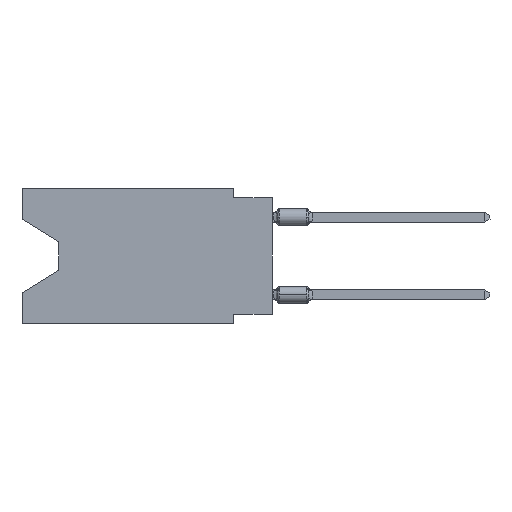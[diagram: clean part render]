
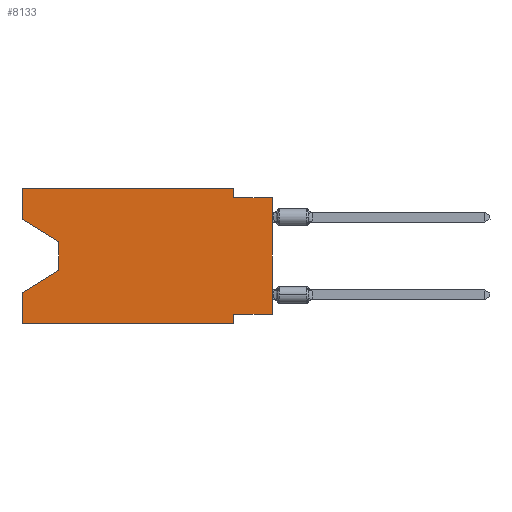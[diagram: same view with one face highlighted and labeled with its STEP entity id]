
A CAD part, left-side view. The second image highlights one B-rep face of the part: STEP entity #8133.
In plain terms, the highlighted planar face has unit normal (-1, 0, 0).
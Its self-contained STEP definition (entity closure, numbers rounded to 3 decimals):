
#111 = DIRECTION ( 'NONE',  ( 0., -1., 0. ) ) ;
#298 = DIRECTION ( 'NONE',  ( 0., 1., 0. ) ) ;
#623 = CARTESIAN_POINT ( 'NONE',  ( 0., 16.383, -2.038 ) ) ;
#681 = CARTESIAN_POINT ( 'NONE',  ( 0., 16.383, -8.89 ) ) ;
#780 = EDGE_CURVE ( 'NONE', #9780, #29481, #25678, .T. ) ;
#806 = CARTESIAN_POINT ( 'NONE',  ( 0., 0., 0. ) ) ;
#1141 = EDGE_CURVE ( 'NONE', #27086, #24400, #24019, .T. ) ;
#2260 = VECTOR ( 'NONE', #25266, 1000. ) ;
#2419 = DIRECTION ( 'NONE',  ( 1., 0., 0. ) ) ;
#2759 = CARTESIAN_POINT ( 'NONE',  ( 0., 0., -8.255 ) ) ;
#2879 = VERTEX_POINT ( 'NONE', #31622 ) ;
#2957 = DIRECTION ( 'NONE',  ( 0., -1., 0. ) ) ;
#3117 = CARTESIAN_POINT ( 'NONE',  ( 0., 16.383, -8.89 ) ) ;
#3632 = DIRECTION ( 'NONE',  ( 0., 0., -1. ) ) ;
#4514 = ORIENTED_EDGE ( 'NONE', *, *, #1141, .T. ) ;
#4577 = VECTOR ( 'NONE', #15066, 1000. ) ;
#5030 = PLANE ( 'NONE',  #8084 ) ;
#5391 = VECTOR ( 'NONE', #6179, 1000. ) ;
#6103 = EDGE_LOOP ( 'NONE', ( #20529, #6624, #4514, #11131, #26470, #29875, #11611, #18943, #21330, #17117, #17707, #25565 ) ) ;
#6111 = VERTEX_POINT ( 'NONE', #17099 ) ;
#6179 = DIRECTION ( 'NONE',  ( 0., 0., 1. ) ) ;
#6624 = ORIENTED_EDGE ( 'NONE', *, *, #27567, .T. ) ;
#7048 = LINE ( 'NONE', #29267, #11227 ) ;
#7839 = LINE ( 'NONE', #681, #12308 ) ;
#8084 = AXIS2_PLACEMENT_3D ( 'NONE', #27078, #2419, #9409 ) ;
#8133 = ADVANCED_FACE ( 'NONE', ( #24633 ), #5030, .F. ) ;
#8614 = CARTESIAN_POINT ( 'NONE',  ( 0., 13.97, -5.385 ) ) ;
#8685 = VECTOR ( 'NONE', #25779, 1000. ) ;
#9052 = DIRECTION ( 'NONE',  ( 0., 0., -1. ) ) ;
#9409 = DIRECTION ( 'NONE',  ( 0., 0., -1. ) ) ;
#9546 = EDGE_CURVE ( 'NONE', #14234, #29481, #7839, .T. ) ;
#9780 = VERTEX_POINT ( 'NONE', #31814 ) ;
#9973 = VERTEX_POINT ( 'NONE', #2759 ) ;
#10060 = EDGE_CURVE ( 'NONE', #9973, #10203, #16207, .T. ) ;
#10203 = VERTEX_POINT ( 'NONE', #31296 ) ;
#10342 = EDGE_CURVE ( 'NONE', #2879, #27320, #22038, .T. ) ;
#11115 = VERTEX_POINT ( 'NONE', #19691 ) ;
#11131 = ORIENTED_EDGE ( 'NONE', *, *, #25760, .F. ) ;
#11227 = VECTOR ( 'NONE', #21647, 1000. ) ;
#11611 = ORIENTED_EDGE ( 'NONE', *, *, #26123, .F. ) ;
#12203 = VECTOR ( 'NONE', #9052, 1000. ) ;
#12308 = VECTOR ( 'NONE', #2957, 1000. ) ;
#13097 = LINE ( 'NONE', #17792, #26980 ) ;
#14200 = VERTEX_POINT ( 'NONE', #15456 ) ;
#14234 = VERTEX_POINT ( 'NONE', #3117 ) ;
#14413 = CARTESIAN_POINT ( 'NONE',  ( 0., 2.54, 0. ) ) ;
#15066 = DIRECTION ( 'NONE',  ( 0., 0., 1. ) ) ;
#15456 = CARTESIAN_POINT ( 'NONE',  ( 0., 13.97, -3.505 ) ) ;
#16207 = LINE ( 'NONE', #806, #8685 ) ;
#16843 = LINE ( 'NONE', #14413, #23573 ) ;
#17099 = CARTESIAN_POINT ( 'NONE',  ( 0., 2.54, 0. ) ) ;
#17117 = ORIENTED_EDGE ( 'NONE', *, *, #27686, .F. ) ;
#17707 = ORIENTED_EDGE ( 'NONE', *, *, #20600, .F. ) ;
#17792 = CARTESIAN_POINT ( 'NONE',  ( 0., 16.383, 0. ) ) ;
#18664 = CARTESIAN_POINT ( 'NONE',  ( 0., 16.383, 0. ) ) ;
#18714 = CARTESIAN_POINT ( 'NONE',  ( 0., 2.54, -8.89 ) ) ;
#18943 = ORIENTED_EDGE ( 'NONE', *, *, #10060, .T. ) ;
#19691 = CARTESIAN_POINT ( 'NONE',  ( 0., 2.54, -0.635 ) ) ;
#20529 = ORIENTED_EDGE ( 'NONE', *, *, #26003, .T. ) ;
#20600 = EDGE_CURVE ( 'NONE', #27320, #6111, #13097, .T. ) ;
#21330 = ORIENTED_EDGE ( 'NONE', *, *, #29175, .F. ) ;
#21647 = DIRECTION ( 'NONE',  ( 0., -1., 0. ) ) ;
#21858 = CARTESIAN_POINT ( 'NONE',  ( 0., 13.97, -3.505 ) ) ;
#21885 = VECTOR ( 'NONE', #3632, 1000. ) ;
#22038 = LINE ( 'NONE', #31939, #4577 ) ;
#22087 = CARTESIAN_POINT ( 'NONE',  ( 0., 2.54, -8.89 ) ) ;
#22210 = LINE ( 'NONE', #623, #2260 ) ;
#22681 = LINE ( 'NONE', #27397, #30221 ) ;
#23573 = VECTOR ( 'NONE', #31919, 1000. ) ;
#24019 = LINE ( 'NONE', #31500, #24998 ) ;
#24400 = VERTEX_POINT ( 'NONE', #30178 ) ;
#24633 = FACE_OUTER_BOUND ( 'NONE', #6103, .T. ) ;
#24998 = VECTOR ( 'NONE', #26293, 1000. ) ;
#25266 = DIRECTION ( 'NONE',  ( 0., -0.855, -0.519 ) ) ;
#25565 = ORIENTED_EDGE ( 'NONE', *, *, #10342, .F. ) ;
#25678 = LINE ( 'NONE', #18714, #21885 ) ;
#25760 = EDGE_CURVE ( 'NONE', #14234, #24400, #25951, .T. ) ;
#25779 = DIRECTION ( 'NONE',  ( 0., 0., 1. ) ) ;
#25951 = LINE ( 'NONE', #18664, #5391 ) ;
#26003 = EDGE_CURVE ( 'NONE', #2879, #14200, #22210, .T. ) ;
#26123 = EDGE_CURVE ( 'NONE', #9973, #9780, #22681, .T. ) ;
#26293 = DIRECTION ( 'NONE',  ( 0., 0.855, -0.519 ) ) ;
#26470 = ORIENTED_EDGE ( 'NONE', *, *, #9546, .T. ) ;
#26980 = VECTOR ( 'NONE', #111, 1000. ) ;
#27078 = CARTESIAN_POINT ( 'NONE',  ( 0., 16.383, 0. ) ) ;
#27086 = VERTEX_POINT ( 'NONE', #8614 ) ;
#27320 = VERTEX_POINT ( 'NONE', #27561 ) ;
#27397 = CARTESIAN_POINT ( 'NONE',  ( 0., 0., -8.255 ) ) ;
#27561 = CARTESIAN_POINT ( 'NONE',  ( 0., 16.383, 0. ) ) ;
#27567 = EDGE_CURVE ( 'NONE', #14200, #27086, #28847, .T. ) ;
#27686 = EDGE_CURVE ( 'NONE', #6111, #11115, #16843, .T. ) ;
#28847 = LINE ( 'NONE', #21858, #12203 ) ;
#29175 = EDGE_CURVE ( 'NONE', #11115, #10203, #7048, .T. ) ;
#29267 = CARTESIAN_POINT ( 'NONE',  ( 0., 0., -0.635 ) ) ;
#29481 = VERTEX_POINT ( 'NONE', #22087 ) ;
#29875 = ORIENTED_EDGE ( 'NONE', *, *, #780, .F. ) ;
#30178 = CARTESIAN_POINT ( 'NONE',  ( 0., 16.383, -6.852 ) ) ;
#30221 = VECTOR ( 'NONE', #298, 1000. ) ;
#31296 = CARTESIAN_POINT ( 'NONE',  ( 0., 0., -0.635 ) ) ;
#31500 = CARTESIAN_POINT ( 'NONE',  ( 0., 13.97, -5.385 ) ) ;
#31622 = CARTESIAN_POINT ( 'NONE',  ( 0., 16.383, -2.038 ) ) ;
#31814 = CARTESIAN_POINT ( 'NONE',  ( 0., 2.54, -8.255 ) ) ;
#31919 = DIRECTION ( 'NONE',  ( 0., 0., -1. ) ) ;
#31939 = CARTESIAN_POINT ( 'NONE',  ( 0., 16.383, 0. ) ) ;
